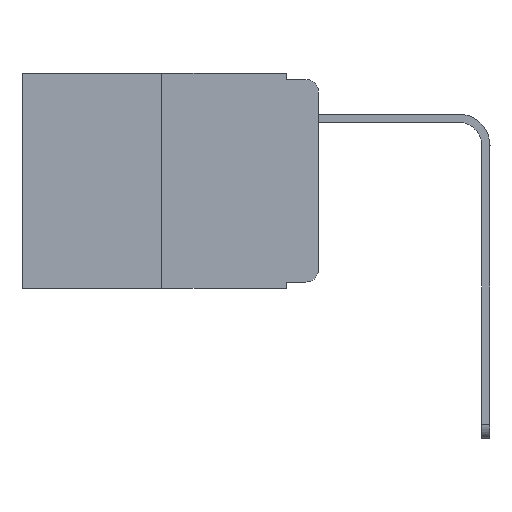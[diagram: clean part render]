
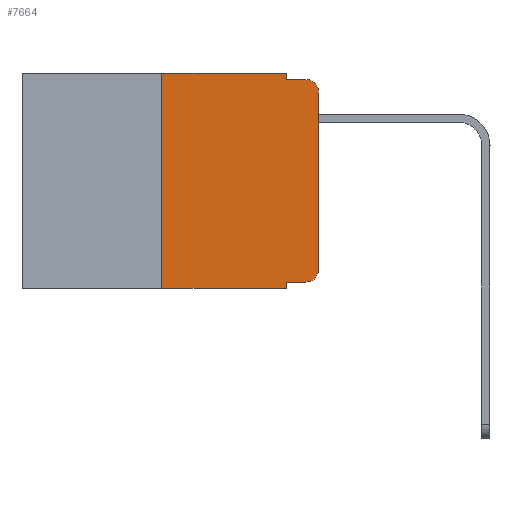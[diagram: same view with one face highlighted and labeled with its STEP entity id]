
A CAD part, left-side view. The second image highlights one B-rep face of the part: STEP entity #7664.
In plain terms, the highlighted planar face has unit normal (-1, 0, 0).
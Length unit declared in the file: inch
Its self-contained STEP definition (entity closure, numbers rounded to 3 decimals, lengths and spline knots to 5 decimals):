
#140 = ORIENTED_EDGE ( 'NONE', *, *, #8420, .F. ) ;
#199 = DIRECTION ( 'NONE',  ( -1., 0., 0. ) ) ;
#254 = CARTESIAN_POINT ( 'NONE',  ( 0., 0., -0.03 ) ) ;
#330 = EDGE_CURVE ( 'NONE', #1823, #5053, #4197, .T. ) ;
#413 = ORIENTED_EDGE ( 'NONE', *, *, #7649, .T. ) ;
#494 = LINE ( 'NONE', #2343, #9516 ) ;
#543 = AXIS2_PLACEMENT_3D ( 'NONE', #9279, #199, #6805 ) ;
#718 = DIRECTION ( 'NONE',  ( 0., -1., 0. ) ) ;
#726 = CARTESIAN_POINT ( 'NONE',  ( 0., 0.051, 0. ) ) ;
#788 = DIRECTION ( 'NONE',  ( 0., -1., 0. ) ) ;
#949 = CARTESIAN_POINT ( 'NONE',  ( 0., 0.051, 0. ) ) ;
#973 = EDGE_CURVE ( 'NONE', #1399, #5837, #1309, .T. ) ;
#1044 = CARTESIAN_POINT ( 'NONE',  ( 0., 0.051, -0.333 ) ) ;
#1165 = DIRECTION ( 'NONE',  ( 0., -1., 0. ) ) ;
#1166 = VERTEX_POINT ( 'NONE', #1530 ) ;
#1211 = VERTEX_POINT ( 'NONE', #6443 ) ;
#1308 = CARTESIAN_POINT ( 'NONE',  ( 0., 0., -0.313 ) ) ;
#1309 = LINE ( 'NONE', #1994, #2758 ) ;
#1399 = VERTEX_POINT ( 'NONE', #5566 ) ;
#1530 = CARTESIAN_POINT ( 'NONE',  ( 0., 0.02, -0.01 ) ) ;
#1780 = CARTESIAN_POINT ( 'NONE',  ( 0., 0.02, -0.313 ) ) ;
#1823 = VERTEX_POINT ( 'NONE', #9472 ) ;
#1845 = ORIENTED_EDGE ( 'NONE', *, *, #330, .T. ) ;
#1994 = CARTESIAN_POINT ( 'NONE',  ( 0., 0.473, 0. ) ) ;
#2019 = VERTEX_POINT ( 'NONE', #7248 ) ;
#2056 = VECTOR ( 'NONE', #7847, 39.37008 ) ;
#2343 = CARTESIAN_POINT ( 'NONE',  ( 0., 0.473, -0.343 ) ) ;
#2360 = EDGE_CURVE ( 'NONE', #5053, #8374, #3507, .T. ) ;
#2408 = VECTOR ( 'NONE', #4691, 39.37008 ) ;
#2471 = VECTOR ( 'NONE', #7088, 39.37008 ) ;
#2675 = EDGE_CURVE ( 'NONE', #10119, #1823, #8739, .T. ) ;
#2685 = DIRECTION ( 'NONE',  ( 0., 0., -1. ) ) ;
#2758 = VECTOR ( 'NONE', #1165, 39.37008 ) ;
#2876 = CARTESIAN_POINT ( 'NONE',  ( 0., 0., 0. ) ) ;
#3108 = CARTESIAN_POINT ( 'NONE',  ( 0., 0.25, 0. ) ) ;
#3507 = LINE ( 'NONE', #2876, #2471 ) ;
#3877 = VECTOR ( 'NONE', #9326, 39.37008 ) ;
#4197 = CIRCLE ( 'NONE', #8516, 0.02 ) ;
#4230 = CARTESIAN_POINT ( 'NONE',  ( 0., 0.473, 0. ) ) ;
#4292 = DIRECTION ( 'NONE',  ( 1., 0., 0. ) ) ;
#4377 = DIRECTION ( 'NONE',  ( -1., 0., 0. ) ) ;
#4623 = ORIENTED_EDGE ( 'NONE', *, *, #2360, .T. ) ;
#4691 = DIRECTION ( 'NONE',  ( 0., 0., 1. ) ) ;
#4792 = CARTESIAN_POINT ( 'NONE',  ( 0., 0.25, -0.343 ) ) ;
#4974 = EDGE_CURVE ( 'NONE', #8694, #1399, #6802, .T. ) ;
#5053 = VERTEX_POINT ( 'NONE', #1308 ) ;
#5106 = EDGE_CURVE ( 'NONE', #5837, #1211, #7475, .T. ) ;
#5566 = CARTESIAN_POINT ( 'NONE',  ( 0., 0.25, 0. ) ) ;
#5837 = VERTEX_POINT ( 'NONE', #949 ) ;
#5884 = CARTESIAN_POINT ( 'NONE',  ( 0., 0.051, 0. ) ) ;
#6032 = DIRECTION ( 'NONE',  ( 0., 0., -1. ) ) ;
#6058 = LINE ( 'NONE', #7695, #2056 ) ;
#6443 = CARTESIAN_POINT ( 'NONE',  ( 0., 0.051, -0.01 ) ) ;
#6465 = VECTOR ( 'NONE', #788, 39.37008 ) ;
#6537 = DIRECTION ( 'NONE',  ( 0., 0., -1. ) ) ;
#6693 = PLANE ( 'NONE',  #8394 ) ;
#6802 = LINE ( 'NONE', #3108, #2408 ) ;
#6805 = DIRECTION ( 'NONE',  ( 0., 0., -1. ) ) ;
#6937 = VECTOR ( 'NONE', #6537, 39.37008 ) ;
#7088 = DIRECTION ( 'NONE',  ( 0., 0., 1. ) ) ;
#7248 = CARTESIAN_POINT ( 'NONE',  ( 0., 0.051, -0.343 ) ) ;
#7459 = CARTESIAN_POINT ( 'NONE',  ( 0., 0.051, -0.333 ) ) ;
#7475 = LINE ( 'NONE', #726, #6937 ) ;
#7649 = EDGE_CURVE ( 'NONE', #8374, #1166, #8612, .T. ) ;
#7664 = ADVANCED_FACE ( 'NONE', ( #9280 ), #6693, .F. ) ;
#7669 = ORIENTED_EDGE ( 'NONE', *, *, #5106, .F. ) ;
#7695 = CARTESIAN_POINT ( 'NONE',  ( 0., 0.051, -0.01 ) ) ;
#7847 = DIRECTION ( 'NONE',  ( 0., -1., 0. ) ) ;
#8374 = VERTEX_POINT ( 'NONE', #254 ) ;
#8394 = AXIS2_PLACEMENT_3D ( 'NONE', #4230, #4292, #2685 ) ;
#8420 = EDGE_CURVE ( 'NONE', #1211, #1166, #6058, .T. ) ;
#8516 = AXIS2_PLACEMENT_3D ( 'NONE', #1780, #4377, #6032 ) ;
#8597 = LINE ( 'NONE', #5884, #3877 ) ;
#8612 = CIRCLE ( 'NONE', #543, 0.02 ) ;
#8694 = VERTEX_POINT ( 'NONE', #4792 ) ;
#8712 = EDGE_CURVE ( 'NONE', #8694, #2019, #494, .T. ) ;
#8739 = LINE ( 'NONE', #7459, #6465 ) ;
#8777 = ORIENTED_EDGE ( 'NONE', *, *, #973, .F. ) ;
#8897 = EDGE_CURVE ( 'NONE', #10119, #2019, #8597, .T. ) ;
#9113 = ORIENTED_EDGE ( 'NONE', *, *, #4974, .F. ) ;
#9279 = CARTESIAN_POINT ( 'NONE',  ( 0., 0.02, -0.03 ) ) ;
#9280 = FACE_OUTER_BOUND ( 'NONE', #10431, .T. ) ;
#9326 = DIRECTION ( 'NONE',  ( 0., 0., -1. ) ) ;
#9472 = CARTESIAN_POINT ( 'NONE',  ( 0., 0.02, -0.333 ) ) ;
#9516 = VECTOR ( 'NONE', #718, 39.37008 ) ;
#9959 = ORIENTED_EDGE ( 'NONE', *, *, #2675, .T. ) ;
#10119 = VERTEX_POINT ( 'NONE', #1044 ) ;
#10431 = EDGE_LOOP ( 'NONE', ( #4623, #413, #140, #7669, #8777, #9113, #10587, #10453, #9959, #1845 ) ) ;
#10453 = ORIENTED_EDGE ( 'NONE', *, *, #8897, .F. ) ;
#10587 = ORIENTED_EDGE ( 'NONE', *, *, #8712, .T. ) ;
